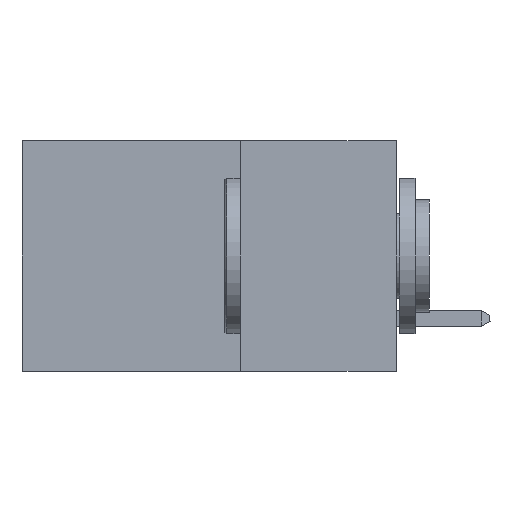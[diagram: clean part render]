
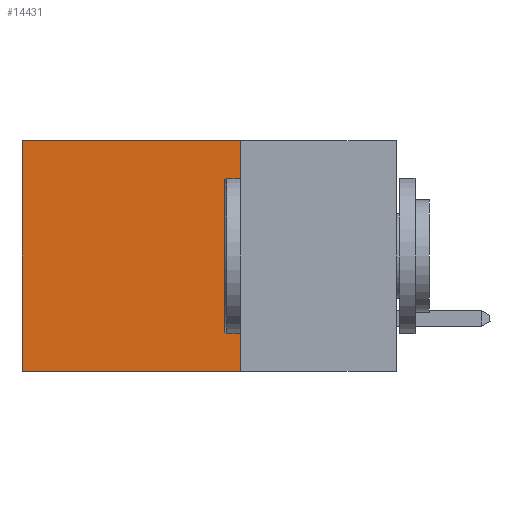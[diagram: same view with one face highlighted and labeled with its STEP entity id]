
A CAD part, left-side view. The second image highlights one B-rep face of the part: STEP entity #14431.
In plain terms, the highlighted planar face has unit normal (-1, 0, 0).
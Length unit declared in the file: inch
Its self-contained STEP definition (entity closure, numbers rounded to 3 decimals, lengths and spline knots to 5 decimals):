
#457 = DIRECTION ( 'NONE',  ( 0., 0., -1. ) ) ;
#856 = VERTEX_POINT ( 'NONE', #8513 ) ;
#970 = DIRECTION ( 'NONE',  ( 0., 1., 0. ) ) ;
#1049 = EDGE_CURVE ( 'NONE', #11192, #2585, #6224, .T. ) ;
#1075 = VECTOR ( 'NONE', #9542, 39.37008 ) ;
#1101 = FACE_OUTER_BOUND ( 'NONE', #13759, .T. ) ;
#1580 = LINE ( 'NONE', #6871, #16779 ) ;
#1756 = VECTOR ( 'NONE', #7395, 39.37008 ) ;
#1778 = PLANE ( 'NONE',  #15424 ) ;
#2585 = VERTEX_POINT ( 'NONE', #18060 ) ;
#4432 = ORIENTED_EDGE ( 'NONE', *, *, #5020, .F. ) ;
#4789 = DIRECTION ( 'NONE',  ( 0., 0., -1. ) ) ;
#4832 = ORIENTED_EDGE ( 'NONE', *, *, #1049, .T. ) ;
#5020 = EDGE_CURVE ( 'NONE', #856, #15892, #9618, .T. ) ;
#5027 = LINE ( 'NONE', #15364, #1075 ) ;
#6224 = LINE ( 'NONE', #9471, #1756 ) ;
#6871 = CARTESIAN_POINT ( 'NONE',  ( 0.298, 0.25, -0.37 ) ) ;
#7395 = DIRECTION ( 'NONE',  ( 0., 0., -1. ) ) ;
#7712 = CARTESIAN_POINT ( 'NONE',  ( 0.298, 0.25, 0. ) ) ;
#8513 = CARTESIAN_POINT ( 'NONE',  ( 0.298, 0.25, 0. ) ) ;
#9162 = VECTOR ( 'NONE', #457, 39.37008 ) ;
#9471 = CARTESIAN_POINT ( 'NONE',  ( 0.298, 0.6, 0. ) ) ;
#9542 = DIRECTION ( 'NONE',  ( 0., 1., 0. ) ) ;
#9618 = LINE ( 'NONE', #16342, #9162 ) ;
#11192 = VERTEX_POINT ( 'NONE', #13127 ) ;
#13127 = CARTESIAN_POINT ( 'NONE',  ( 0.298, 0.6, 0. ) ) ;
#13405 = ORIENTED_EDGE ( 'NONE', *, *, #15267, .T. ) ;
#13646 = DIRECTION ( 'NONE',  ( 1., 0., 0. ) ) ;
#13759 = EDGE_LOOP ( 'NONE', ( #4832, #18813, #4432, #13405 ) ) ;
#14159 = CARTESIAN_POINT ( 'NONE',  ( 0.298, 0.25, -0.37 ) ) ;
#14431 = ADVANCED_FACE ( 'NONE', ( #1101 ), #1778, .F. ) ;
#15267 = EDGE_CURVE ( 'NONE', #856, #11192, #5027, .T. ) ;
#15364 = CARTESIAN_POINT ( 'NONE',  ( 0.298, 0.25, 0. ) ) ;
#15424 = AXIS2_PLACEMENT_3D ( 'NONE', #7712, #13646, #4789 ) ;
#15892 = VERTEX_POINT ( 'NONE', #14159 ) ;
#16342 = CARTESIAN_POINT ( 'NONE',  ( 0.298, 0.25, 0. ) ) ;
#16603 = EDGE_CURVE ( 'NONE', #15892, #2585, #1580, .T. ) ;
#16779 = VECTOR ( 'NONE', #970, 39.37008 ) ;
#18060 = CARTESIAN_POINT ( 'NONE',  ( 0.298, 0.6, -0.37 ) ) ;
#18813 = ORIENTED_EDGE ( 'NONE', *, *, #16603, .F. ) ;
